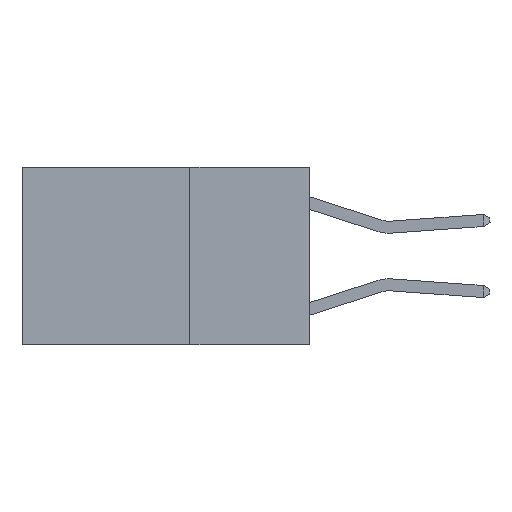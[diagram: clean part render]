
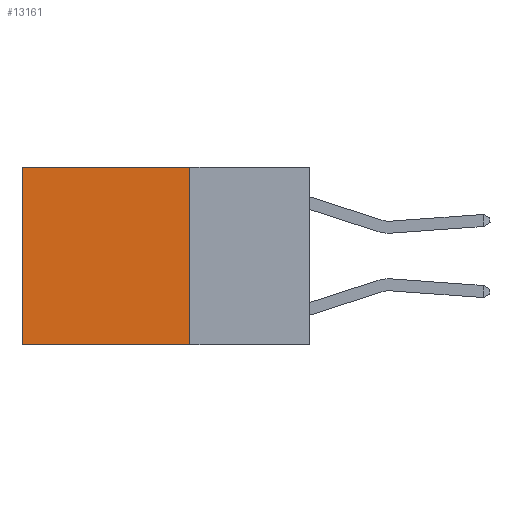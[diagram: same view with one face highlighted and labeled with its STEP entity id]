
A CAD part, left-side view. The second image highlights one B-rep face of the part: STEP entity #13161.
In plain terms, the highlighted planar face has unit normal (-1, 0, 0).
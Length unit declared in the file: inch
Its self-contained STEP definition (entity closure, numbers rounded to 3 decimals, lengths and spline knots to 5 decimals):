
#92 = CARTESIAN_POINT ( 'NONE',  ( 0.2625, 0.25, -0.37 ) ) ;
#383 = DIRECTION ( 'NONE',  ( 0., 1., 0. ) ) ;
#925 = VERTEX_POINT ( 'NONE', #11097 ) ;
#1184 = DIRECTION ( 'NONE',  ( 0., 1., 0. ) ) ;
#1296 = VECTOR ( 'NONE', #3046, 39.37008 ) ;
#1732 = VECTOR ( 'NONE', #8170, 39.37008 ) ;
#1891 = ORIENTED_EDGE ( 'NONE', *, *, #3620, .F. ) ;
#2241 = VERTEX_POINT ( 'NONE', #3130 ) ;
#3046 = DIRECTION ( 'NONE',  ( 0., 0., -1. ) ) ;
#3055 = LINE ( 'NONE', #7495, #8422 ) ;
#3130 = CARTESIAN_POINT ( 'NONE',  ( 0.2625, 0.25, 0. ) ) ;
#3138 = CARTESIAN_POINT ( 'NONE',  ( 0.2625, 0.25, 0. ) ) ;
#3620 = EDGE_CURVE ( 'NONE', #5363, #925, #3055, .T. ) ;
#4146 = EDGE_CURVE ( 'NONE', #2241, #4473, #7457, .T. ) ;
#4449 = ORIENTED_EDGE ( 'NONE', *, *, #4146, .T. ) ;
#4473 = VERTEX_POINT ( 'NONE', #4749 ) ;
#4749 = CARTESIAN_POINT ( 'NONE',  ( 0.2625, 0.6, 0. ) ) ;
#4763 = LINE ( 'NONE', #3138, #1732 ) ;
#4788 = VECTOR ( 'NONE', #1184, 39.37008 ) ;
#5242 = CARTESIAN_POINT ( 'NONE',  ( 0.2625, 0.25, 0. ) ) ;
#5363 = VERTEX_POINT ( 'NONE', #92 ) ;
#5592 = AXIS2_PLACEMENT_3D ( 'NONE', #7923, #5959, #13044 ) ;
#5764 = EDGE_LOOP ( 'NONE', ( #8721, #1891, #9656, #4449 ) ) ;
#5959 = DIRECTION ( 'NONE',  ( 1., 0., 0. ) ) ;
#6447 = EDGE_CURVE ( 'NONE', #4473, #925, #12432, .T. ) ;
#6975 = FACE_OUTER_BOUND ( 'NONE', #5764, .T. ) ;
#7457 = LINE ( 'NONE', #5242, #4788 ) ;
#7495 = CARTESIAN_POINT ( 'NONE',  ( 0.2625, 0.25, -0.37 ) ) ;
#7923 = CARTESIAN_POINT ( 'NONE',  ( 0.2625, 0.25, 0. ) ) ;
#8170 = DIRECTION ( 'NONE',  ( 0., 0., -1. ) ) ;
#8383 = EDGE_CURVE ( 'NONE', #2241, #5363, #4763, .T. ) ;
#8422 = VECTOR ( 'NONE', #383, 39.37008 ) ;
#8721 = ORIENTED_EDGE ( 'NONE', *, *, #6447, .T. ) ;
#9656 = ORIENTED_EDGE ( 'NONE', *, *, #8383, .F. ) ;
#9983 = PLANE ( 'NONE',  #5592 ) ;
#10150 = CARTESIAN_POINT ( 'NONE',  ( 0.2625, 0.6, 0. ) ) ;
#11097 = CARTESIAN_POINT ( 'NONE',  ( 0.2625, 0.6, -0.37 ) ) ;
#12432 = LINE ( 'NONE', #10150, #1296 ) ;
#13044 = DIRECTION ( 'NONE',  ( 0., 0., -1. ) ) ;
#13161 = ADVANCED_FACE ( 'NONE', ( #6975 ), #9983, .F. ) ;
